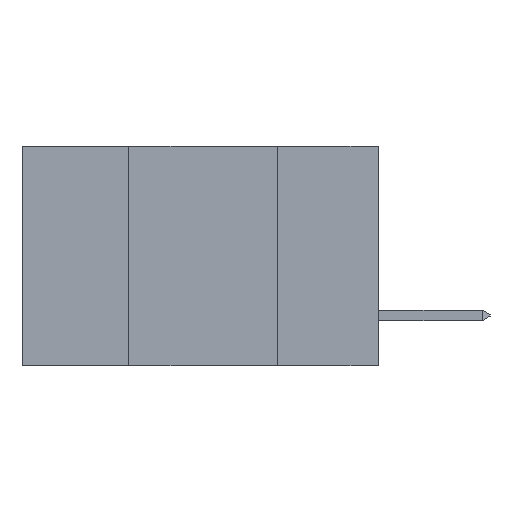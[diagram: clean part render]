
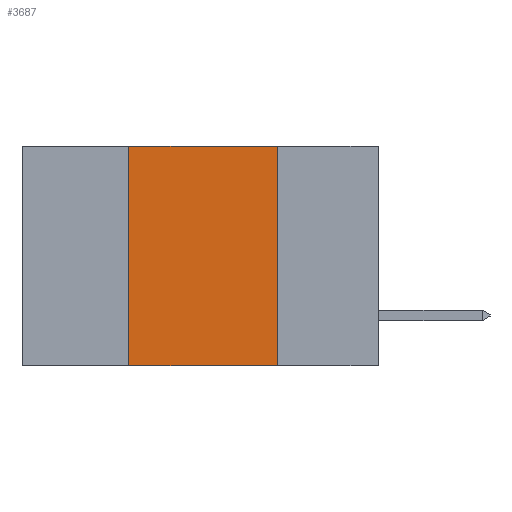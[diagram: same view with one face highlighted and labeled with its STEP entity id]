
A CAD part, left-side view. The second image highlights one B-rep face of the part: STEP entity #3687.
In plain terms, the highlighted planar face has unit normal (-1, 0, 0).
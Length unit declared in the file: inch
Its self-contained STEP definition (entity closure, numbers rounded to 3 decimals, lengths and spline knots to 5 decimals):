
#105 = LINE ( 'NONE', #6293, #9904 ) ;
#133 = CARTESIAN_POINT ( 'NONE',  ( 0., 0.6, 0. ) ) ;
#212 = VECTOR ( 'NONE', #6422, 39.37008 ) ;
#334 = VECTOR ( 'NONE', #1725, 39.37008 ) ;
#450 = CARTESIAN_POINT ( 'NONE',  ( 0., 0.42, 0. ) ) ;
#650 = CARTESIAN_POINT ( 'NONE',  ( 0., 0.17, -0.37 ) ) ;
#917 = PLANE ( 'NONE',  #8925 ) ;
#1725 = DIRECTION ( 'NONE',  ( 0., -1., 0. ) ) ;
#1943 = DIRECTION ( 'NONE',  ( 1., 0., 0. ) ) ;
#2123 = EDGE_CURVE ( 'NONE', #3404, #5801, #10329, .T. ) ;
#2975 = LINE ( 'NONE', #10124, #334 ) ;
#3131 = CARTESIAN_POINT ( 'NONE',  ( 0., 0.17, 0. ) ) ;
#3404 = VERTEX_POINT ( 'NONE', #450 ) ;
#3612 = ORIENTED_EDGE ( 'NONE', *, *, #4052, .F. ) ;
#3687 = ADVANCED_FACE ( 'NONE', ( #7728 ), #917, .F. ) ;
#3904 = ORIENTED_EDGE ( 'NONE', *, *, #10483, .F. ) ;
#4052 = EDGE_CURVE ( 'NONE', #5801, #4581, #10000, .T. ) ;
#4490 = EDGE_LOOP ( 'NONE', ( #3612, #11004, #3904, #6406 ) ) ;
#4581 = VERTEX_POINT ( 'NONE', #11748 ) ;
#5540 = EDGE_CURVE ( 'NONE', #6945, #4581, #2975, .T. ) ;
#5801 = VERTEX_POINT ( 'NONE', #3131 ) ;
#6293 = CARTESIAN_POINT ( 'NONE',  ( 0., 0.42, -0.37 ) ) ;
#6406 = ORIENTED_EDGE ( 'NONE', *, *, #5540, .T. ) ;
#6422 = DIRECTION ( 'NONE',  ( 0., 0., -1. ) ) ;
#6945 = VERTEX_POINT ( 'NONE', #9536 ) ;
#7620 = CARTESIAN_POINT ( 'NONE',  ( 0., 0.6, 0. ) ) ;
#7728 = FACE_OUTER_BOUND ( 'NONE', #4490, .T. ) ;
#7911 = VECTOR ( 'NONE', #12144, 39.37008 ) ;
#8527 = DIRECTION ( 'NONE',  ( 0., 0., -1. ) ) ;
#8925 = AXIS2_PLACEMENT_3D ( 'NONE', #7620, #1943, #8527 ) ;
#9049 = DIRECTION ( 'NONE',  ( 0., 0., 1. ) ) ;
#9536 = CARTESIAN_POINT ( 'NONE',  ( 0., 0.42, -0.37 ) ) ;
#9904 = VECTOR ( 'NONE', #9049, 39.37008 ) ;
#10000 = LINE ( 'NONE', #650, #212 ) ;
#10124 = CARTESIAN_POINT ( 'NONE',  ( 0., 0.6, -0.37 ) ) ;
#10329 = LINE ( 'NONE', #133, #7911 ) ;
#10483 = EDGE_CURVE ( 'NONE', #6945, #3404, #105, .T. ) ;
#11004 = ORIENTED_EDGE ( 'NONE', *, *, #2123, .F. ) ;
#11748 = CARTESIAN_POINT ( 'NONE',  ( 0., 0.17, -0.37 ) ) ;
#12144 = DIRECTION ( 'NONE',  ( 0., -1., 0. ) ) ;
